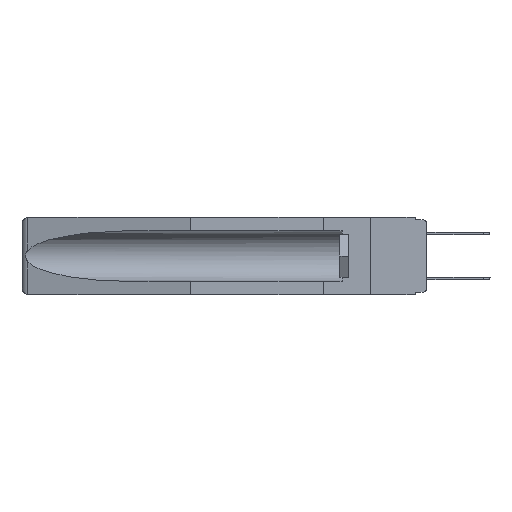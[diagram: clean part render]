
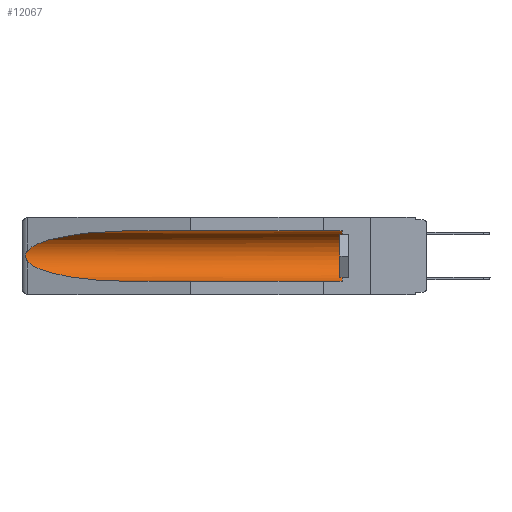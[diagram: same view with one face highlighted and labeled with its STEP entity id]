
A CAD part, left-side view. The second image highlights one B-rep face of the part: STEP entity #12067.
In plain terms, the highlighted cylindrical face has radius 2.857 mm (diameter 5.715 mm), a partial arc.
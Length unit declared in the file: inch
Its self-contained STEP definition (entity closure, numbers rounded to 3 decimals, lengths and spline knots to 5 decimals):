
#90 = CARTESIAN_POINT ( 'NONE',  ( 0.26597, 1.52961, -0.15275 ) ) ;
#164 = CARTESIAN_POINT ( 'NONE',  ( 0.26537, 1.52718, -0.14972 ) ) ;
#310 = FACE_OUTER_BOUND ( 'NONE', #14178, .T. ) ;
#1273 = CARTESIAN_POINT ( 'NONE',  ( 0.21114, 1.30732, -0.059 ) ) ;
#1838 = CARTESIAN_POINT ( 'NONE',  ( 0.2675, 1.53308, -0.17534 ) ) ;
#2128 = CARTESIAN_POINT ( 'NONE',  ( 0.155, -0.30754, -0.1715 ) ) ;
#2310 = EDGE_CURVE ( 'NONE', #5810, #20235, #24221, .T. ) ;
#3035 = EDGE_CURVE ( 'NONE', #18105, #22726, #9163, .T. ) ;
#3512 = CARTESIAN_POINT ( 'NONE',  ( 0.26537, 1.52718, -0.19328 ) ) ;
#3846 = ORIENTED_EDGE ( 'NONE', *, *, #2310, .T. ) ;
#4040 = CARTESIAN_POINT ( 'NONE',  ( 0.155, -0.30754, -0.284 ) ) ;
#4218 = ORIENTED_EDGE ( 'NONE', *, *, #20014, .T. ) ;
#4258 = EDGE_CURVE ( 'NONE', #18105, #19616, #10885, .T. ) ;
#4530 = DIRECTION ( 'NONE',  ( 0., 1., 0. ) ) ;
#5202 = CARTESIAN_POINT ( 'NONE',  ( 0.155, 0.126, -0.1715 ) ) ;
#5810 = VERTEX_POINT ( 'NONE', #22001 ) ;
#6997 = CARTESIAN_POINT ( 'NONE',  ( 0.155, 1.07973, -0.284 ) ) ;
#7024 = CARTESIAN_POINT ( 'NONE',  ( 0.155, 1.07973, -0.059 ) ) ;
#7082 = VECTOR ( 'NONE', #20683, 39.37008 ) ;
#7368 = ORIENTED_EDGE ( 'NONE', *, *, #3035, .F. ) ;
#9163 = LINE ( 'NONE', #4040, #7082 ) ;
#9644 = AXIS2_PLACEMENT_3D ( 'NONE', #5202, #10918, #12722 ) ;
#9694 = VERTEX_POINT ( 'NONE', #15568 ) ;
#10885 = CIRCLE ( 'NONE', #9644, 0.1125 ) ;
#10918 = DIRECTION ( 'NONE',  ( 0., -1., 0. ) ) ;
#11779 = AXIS2_PLACEMENT_3D ( 'NONE', #2128, #15350, #17301 ) ;
#11897 = CARTESIAN_POINT ( 'NONE',  ( 0.155, -0.30754, -0.059 ) ) ;
#12067 = ADVANCED_FACE ( 'NONE', ( #310 ), #12508, .F. ) ;
#12508 = CYLINDRICAL_SURFACE ( 'NONE', #11779, 0.1125 ) ;
#12722 = DIRECTION ( 'NONE',  ( 0., 0., 1. ) ) ;
#13398 = CARTESIAN_POINT ( 'NONE',  ( 0.26537, 1.52718, -0.19328 ) ) ;
#13931 =( BOUNDED_CURVE ( )  B_SPLINE_CURVE ( 3, ( #23690, #21765, #16169, #19935 ),
 .UNSPECIFIED., .F., .F. ) 
 B_SPLINE_CURVE_WITH_KNOTS ( ( 4, 4 ),
 ( 0.1948, 1.5708 ),
 .UNSPECIFIED. ) 
 CURVE ( )  GEOMETRIC_REPRESENTATION_ITEM ( )  RATIONAL_B_SPLINE_CURVE ( ( 1., 0.848, 0.848, 1. ) ) 
 REPRESENTATION_ITEM ( '' )  );
#14178 = EDGE_LOOP ( 'NONE', ( #22042, #3846, #17598, #7368, #24300, #4218 ) ) ;
#15350 = DIRECTION ( 'NONE',  ( 0., 1., 0. ) ) ;
#15568 = CARTESIAN_POINT ( 'NONE',  ( 0.155, 1.07973, -0.059 ) ) ;
#15726 = CARTESIAN_POINT ( 'NONE',  ( 0.155, 0.126, -0.284 ) ) ;
#16169 = CARTESIAN_POINT ( 'NONE',  ( 0.21114, 1.30732, -0.284 ) ) ;
#16382 = CARTESIAN_POINT ( 'NONE',  ( 0.25451, 1.48313, -0.09465 ) ) ;
#16762 = CARTESIAN_POINT ( 'NONE',  ( 0.2673, 1.53269, -0.17917 ) ) ;
#17082 = CARTESIAN_POINT ( 'NONE',  ( 0.26597, 1.5296, -0.19026 ) ) ;
#17301 = DIRECTION ( 'NONE',  ( 0., 0., 1. ) ) ;
#17598 = ORIENTED_EDGE ( 'NONE', *, *, #19430, .T. ) ;
#18077 = VECTOR ( 'NONE', #4530, 39.37008 ) ;
#18105 = VERTEX_POINT ( 'NONE', #15726 ) ;
#18803 = CARTESIAN_POINT ( 'NONE',  ( 0.26654, 1.53092, -0.15636 ) ) ;
#19430 = EDGE_CURVE ( 'NONE', #20235, #22726, #13931, .T. ) ;
#19616 = VERTEX_POINT ( 'NONE', #20350 ) ;
#19935 = CARTESIAN_POINT ( 'NONE',  ( 0.155, 1.07973, -0.284 ) ) ;
#20014 = EDGE_CURVE ( 'NONE', #19616, #9694, #20466, .T. ) ;
#20235 = VERTEX_POINT ( 'NONE', #3512 ) ;
#20350 = CARTESIAN_POINT ( 'NONE',  ( 0.155, 0.126, -0.059 ) ) ;
#20466 = LINE ( 'NONE', #11897, #18077 ) ;
#20683 = DIRECTION ( 'NONE',  ( 0., 1., 0. ) ) ;
#20715 = CARTESIAN_POINT ( 'NONE',  ( 0.2675, 1.53308, -0.16763 ) ) ;
#21765 = CARTESIAN_POINT ( 'NONE',  ( 0.25451, 1.48313, -0.24835 ) ) ;
#22001 = CARTESIAN_POINT ( 'NONE',  ( 0.26537, 1.52718, -0.14972 ) ) ;
#22006 = EDGE_CURVE ( 'NONE', #9694, #5810, #22375, .T. ) ;
#22042 = ORIENTED_EDGE ( 'NONE', *, *, #22006, .T. ) ;
#22375 =( BOUNDED_CURVE ( )  B_SPLINE_CURVE ( 3, ( #7024, #1273, #16382, #23984 ),
 .UNSPECIFIED., .F., .F. ) 
 B_SPLINE_CURVE_WITH_KNOTS ( ( 4, 4 ),
 ( 4.71239, 6.08839 ),
 .UNSPECIFIED. ) 
 CURVE ( )  GEOMETRIC_REPRESENTATION_ITEM ( )  RATIONAL_B_SPLINE_CURVE ( ( 1., 0.848, 0.848, 1. ) ) 
 REPRESENTATION_ITEM ( '' )  );
#22543 = CARTESIAN_POINT ( 'NONE',  ( 0.2673, 1.5327, -0.16383 ) ) ;
#22726 = VERTEX_POINT ( 'NONE', #6997 ) ;
#23690 = CARTESIAN_POINT ( 'NONE',  ( 0.26537, 1.52718, -0.19328 ) ) ;
#23984 = CARTESIAN_POINT ( 'NONE',  ( 0.26537, 1.52718, -0.14972 ) ) ;
#24221 = B_SPLINE_CURVE_WITH_KNOTS ( 'NONE', 3,
 ( #164, #90, #18803, #22543, #20715, #1838, #16762, #24384, #17082, #13398 ),
 .UNSPECIFIED., .F., .F.,
 ( 4, 2, 2, 2, 4 ),
 ( 0., 0.00029, 0.00058, 0.00087, 0.00117 ),
 .UNSPECIFIED. ) ;
#24300 = ORIENTED_EDGE ( 'NONE', *, *, #4258, .T. ) ;
#24384 = CARTESIAN_POINT ( 'NONE',  ( 0.26655, 1.53094, -0.18657 ) ) ;
